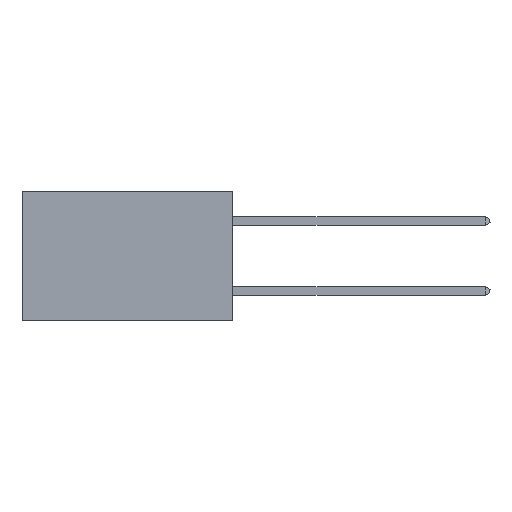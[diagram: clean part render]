
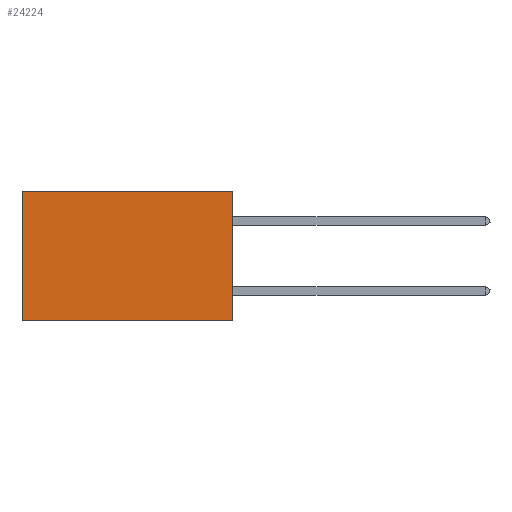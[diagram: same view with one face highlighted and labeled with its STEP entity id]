
A CAD part, left-side view. The second image highlights one B-rep face of the part: STEP entity #24224.
In plain terms, the highlighted planar face has unit normal (-1, 0, 0).
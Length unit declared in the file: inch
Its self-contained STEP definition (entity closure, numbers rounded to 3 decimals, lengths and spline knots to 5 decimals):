
#1003 = PLANE ( 'NONE',  #17333 ) ;
#1461 = LINE ( 'NONE', #8132, #12686 ) ;
#2553 = DIRECTION ( 'NONE',  ( 0., 0., -1. ) ) ;
#3780 = ORIENTED_EDGE ( 'NONE', *, *, #21256, .F. ) ;
#4271 = ORIENTED_EDGE ( 'NONE', *, *, #11567, .F. ) ;
#4430 = EDGE_CURVE ( 'NONE', #4941, #7810, #1461, .T. ) ;
#4941 = VERTEX_POINT ( 'NONE', #20508 ) ;
#5080 = CARTESIAN_POINT ( 'NONE',  ( 0.2875, 0., -0.37 ) ) ;
#5563 = CARTESIAN_POINT ( 'NONE',  ( 0.2875, 0., 0. ) ) ;
#5904 = VECTOR ( 'NONE', #2553, 39.37008 ) ;
#6436 = DIRECTION ( 'NONE',  ( 0., 1., 0. ) ) ;
#6597 = ORIENTED_EDGE ( 'NONE', *, *, #14266, .T. ) ;
#6621 = CARTESIAN_POINT ( 'NONE',  ( 0.2875, 0., 0. ) ) ;
#7439 = CARTESIAN_POINT ( 'NONE',  ( 0.2875, 0.6, -0.37 ) ) ;
#7803 = VERTEX_POINT ( 'NONE', #5080 ) ;
#7810 = VERTEX_POINT ( 'NONE', #7439 ) ;
#7817 = DIRECTION ( 'NONE',  ( 0., 0., -1. ) ) ;
#8132 = CARTESIAN_POINT ( 'NONE',  ( 0.2875, 0.6, 0. ) ) ;
#11567 = EDGE_CURVE ( 'NONE', #22690, #7803, #17617, .T. ) ;
#12529 = DIRECTION ( 'NONE',  ( 0., 1., 0. ) ) ;
#12686 = VECTOR ( 'NONE', #23224, 39.37008 ) ;
#13665 = LINE ( 'NONE', #21607, #24265 ) ;
#14266 = EDGE_CURVE ( 'NONE', #22690, #4941, #25992, .T. ) ;
#17333 = AXIS2_PLACEMENT_3D ( 'NONE', #5563, #20792, #7817 ) ;
#17617 = LINE ( 'NONE', #20106, #5904 ) ;
#20106 = CARTESIAN_POINT ( 'NONE',  ( 0.2875, 0., 0. ) ) ;
#20291 = EDGE_LOOP ( 'NONE', ( #21690, #3780, #4271, #6597 ) ) ;
#20386 = VECTOR ( 'NONE', #12529, 39.37008 ) ;
#20508 = CARTESIAN_POINT ( 'NONE',  ( 0.2875, 0.6, 0. ) ) ;
#20792 = DIRECTION ( 'NONE',  ( 1., 0., 0. ) ) ;
#21029 = CARTESIAN_POINT ( 'NONE',  ( 0.2875, 0., 0. ) ) ;
#21256 = EDGE_CURVE ( 'NONE', #7803, #7810, #13665, .T. ) ;
#21607 = CARTESIAN_POINT ( 'NONE',  ( 0.2875, 0., -0.37 ) ) ;
#21690 = ORIENTED_EDGE ( 'NONE', *, *, #4430, .T. ) ;
#22690 = VERTEX_POINT ( 'NONE', #6621 ) ;
#23224 = DIRECTION ( 'NONE',  ( 0., 0., -1. ) ) ;
#24224 = ADVANCED_FACE ( 'NONE', ( #27663 ), #1003, .F. ) ;
#24265 = VECTOR ( 'NONE', #6436, 39.37008 ) ;
#25992 = LINE ( 'NONE', #21029, #20386 ) ;
#27663 = FACE_OUTER_BOUND ( 'NONE', #20291, .T. ) ;
